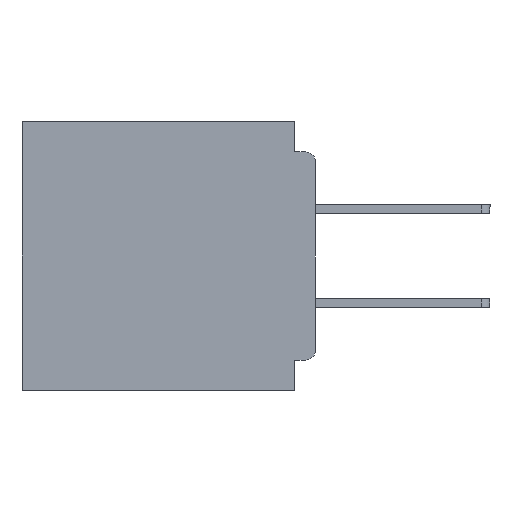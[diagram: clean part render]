
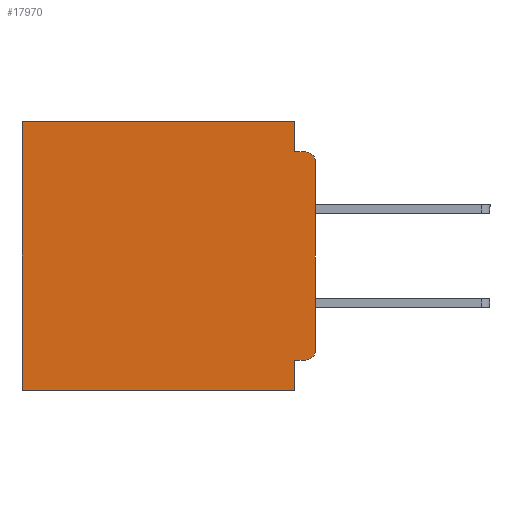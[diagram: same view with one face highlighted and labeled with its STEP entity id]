
A CAD part, left-side view. The second image highlights one B-rep face of the part: STEP entity #17970.
In plain terms, the highlighted planar face has unit normal (-1, 0, 0).
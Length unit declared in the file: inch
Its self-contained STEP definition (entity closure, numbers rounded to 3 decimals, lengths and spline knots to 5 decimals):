
#68 = CARTESIAN_POINT ( 'NONE',  ( 0.3, 0.031, -0.355 ) ) ;
#694 = LINE ( 'NONE', #2508, #24559 ) ;
#912 = LINE ( 'NONE', #37782, #33319 ) ;
#1631 = AXIS2_PLACEMENT_3D ( 'NONE', #31240, #11961, #34483 ) ;
#1900 = LINE ( 'NONE', #38308, #34336 ) ;
#2508 = CARTESIAN_POINT ( 'NONE',  ( 0.3, 0., -0.045 ) ) ;
#3095 = DIRECTION ( 'NONE',  ( 0., 0., -1. ) ) ;
#3319 = EDGE_LOOP ( 'NONE', ( #9351, #16929, #15928, #27590, #31103, #40798, #6917, #16625, #17623, #4882 ) ) ;
#3623 = EDGE_CURVE ( 'NONE', #22119, #36767, #1900, .T. ) ;
#3862 = VERTEX_POINT ( 'NONE', #19398 ) ;
#4189 = DIRECTION ( 'NONE',  ( 0., 0., -1. ) ) ;
#4882 = ORIENTED_EDGE ( 'NONE', *, *, #39380, .T. ) ;
#5830 = VECTOR ( 'NONE', #29609, 39.37008 ) ;
#6917 = ORIENTED_EDGE ( 'NONE', *, *, #3623, .F. ) ;
#7149 = VERTEX_POINT ( 'NONE', #9080 ) ;
#7161 = VECTOR ( 'NONE', #3095, 39.37008 ) ;
#7406 = DIRECTION ( 'NONE',  ( 0., 1., 0. ) ) ;
#8668 = LINE ( 'NONE', #23738, #32377 ) ;
#8686 = CARTESIAN_POINT ( 'NONE',  ( 0.3, 0., -0.4 ) ) ;
#9080 = CARTESIAN_POINT ( 'NONE',  ( 0.3, 0.015, -0.045 ) ) ;
#9348 = DIRECTION ( 'NONE',  ( -1., 0., 0. ) ) ;
#9351 = ORIENTED_EDGE ( 'NONE', *, *, #19699, .F. ) ;
#10685 = VECTOR ( 'NONE', #21837, 39.37008 ) ;
#11367 = VERTEX_POINT ( 'NONE', #31036 ) ;
#11713 = LINE ( 'NONE', #8686, #10685 ) ;
#11961 = DIRECTION ( 'NONE',  ( -1., 0., 0. ) ) ;
#12070 = CIRCLE ( 'NONE', #19144, 0.015 ) ;
#12273 = DIRECTION ( 'NONE',  ( 0., -1., 0. ) ) ;
#12663 = EDGE_CURVE ( 'NONE', #40496, #7149, #12070, .T. ) ;
#13006 = VERTEX_POINT ( 'NONE', #33566 ) ;
#13860 = VECTOR ( 'NONE', #19339, 39.37008 ) ;
#14357 = FACE_OUTER_BOUND ( 'NONE', #3319, .T. ) ;
#14485 = LINE ( 'NONE', #39198, #5830 ) ;
#14874 = LINE ( 'NONE', #16074, #13860 ) ;
#15259 = DIRECTION ( 'NONE',  ( 0., 0., -1. ) ) ;
#15794 = LINE ( 'NONE', #25791, #7161 ) ;
#15928 = ORIENTED_EDGE ( 'NONE', *, *, #33443, .F. ) ;
#16074 = CARTESIAN_POINT ( 'NONE',  ( 0.3, 0., 0. ) ) ;
#16625 = ORIENTED_EDGE ( 'NONE', *, *, #29114, .F. ) ;
#16929 = ORIENTED_EDGE ( 'NONE', *, *, #12663, .T. ) ;
#17156 = VERTEX_POINT ( 'NONE', #26080 ) ;
#17358 = DIRECTION ( 'NONE',  ( 0., 1., 0. ) ) ;
#17489 = CARTESIAN_POINT ( 'NONE',  ( 0.3, 0., -0.06 ) ) ;
#17623 = ORIENTED_EDGE ( 'NONE', *, *, #25612, .F. ) ;
#17970 = ADVANCED_FACE ( 'NONE', ( #14357 ), #20413, .F. ) ;
#19144 = AXIS2_PLACEMENT_3D ( 'NONE', #28670, #9348, #31923 ) ;
#19210 = CARTESIAN_POINT ( 'NONE',  ( 0.3, 0.031, 0. ) ) ;
#19339 = DIRECTION ( 'NONE',  ( 0., 1., 0. ) ) ;
#19398 = CARTESIAN_POINT ( 'NONE',  ( 0.3, 0.015, -0.355 ) ) ;
#19699 = EDGE_CURVE ( 'NONE', #40496, #11367, #11713, .T. ) ;
#20413 = PLANE ( 'NONE',  #26937 ) ;
#21837 = DIRECTION ( 'NONE',  ( 0., 0., -1. ) ) ;
#22119 = VERTEX_POINT ( 'NONE', #28869 ) ;
#23502 = CIRCLE ( 'NONE', #1631, 0.015 ) ;
#23652 = DIRECTION ( 'NONE',  ( 1., 0., 0. ) ) ;
#23738 = CARTESIAN_POINT ( 'NONE',  ( 0.3, 0., -0.355 ) ) ;
#24096 = EDGE_CURVE ( 'NONE', #31267, #13006, #14874, .T. ) ;
#24559 = VECTOR ( 'NONE', #12273, 39.37008 ) ;
#25612 = EDGE_CURVE ( 'NONE', #3862, #39598, #8668, .T. ) ;
#25791 = CARTESIAN_POINT ( 'NONE',  ( 0.3, 0.437, -0.4 ) ) ;
#26080 = CARTESIAN_POINT ( 'NONE',  ( 0.3, 0.031, -0.045 ) ) ;
#26937 = AXIS2_PLACEMENT_3D ( 'NONE', #36427, #23652, #4189 ) ;
#27590 = ORIENTED_EDGE ( 'NONE', *, *, #35582, .F. ) ;
#28670 = CARTESIAN_POINT ( 'NONE',  ( 0.3, 0.015, -0.06 ) ) ;
#28869 = CARTESIAN_POINT ( 'NONE',  ( 0.3, 0.031, -0.4 ) ) ;
#29114 = EDGE_CURVE ( 'NONE', #39598, #22119, #14485, .T. ) ;
#29609 = DIRECTION ( 'NONE',  ( 0., 0., -1. ) ) ;
#31036 = CARTESIAN_POINT ( 'NONE',  ( 0.3, 0., -0.34 ) ) ;
#31103 = ORIENTED_EDGE ( 'NONE', *, *, #24096, .T. ) ;
#31240 = CARTESIAN_POINT ( 'NONE',  ( 0.3, 0.015, -0.34 ) ) ;
#31267 = VERTEX_POINT ( 'NONE', #19210 ) ;
#31923 = DIRECTION ( 'NONE',  ( 0., 0., -1. ) ) ;
#32377 = VECTOR ( 'NONE', #17358, 39.37008 ) ;
#33319 = VECTOR ( 'NONE', #15259, 39.37008 ) ;
#33443 = EDGE_CURVE ( 'NONE', #17156, #7149, #694, .T. ) ;
#33566 = CARTESIAN_POINT ( 'NONE',  ( 0.3, 0.437, 0. ) ) ;
#34157 = CARTESIAN_POINT ( 'NONE',  ( 0.3, 0.437, -0.4 ) ) ;
#34336 = VECTOR ( 'NONE', #7406, 39.37008 ) ;
#34483 = DIRECTION ( 'NONE',  ( 0., 0., -1. ) ) ;
#35582 = EDGE_CURVE ( 'NONE', #31267, #17156, #912, .T. ) ;
#36427 = CARTESIAN_POINT ( 'NONE',  ( 0.3, 0., -0.4 ) ) ;
#36767 = VERTEX_POINT ( 'NONE', #34157 ) ;
#37782 = CARTESIAN_POINT ( 'NONE',  ( 0.3, 0.031, 0. ) ) ;
#38308 = CARTESIAN_POINT ( 'NONE',  ( 0.3, 0., -0.4 ) ) ;
#39198 = CARTESIAN_POINT ( 'NONE',  ( 0.3, 0.031, -0.4 ) ) ;
#39380 = EDGE_CURVE ( 'NONE', #3862, #11367, #23502, .T. ) ;
#39598 = VERTEX_POINT ( 'NONE', #68 ) ;
#40496 = VERTEX_POINT ( 'NONE', #17489 ) ;
#40798 = ORIENTED_EDGE ( 'NONE', *, *, #41631, .T. ) ;
#41631 = EDGE_CURVE ( 'NONE', #13006, #36767, #15794, .T. ) ;
